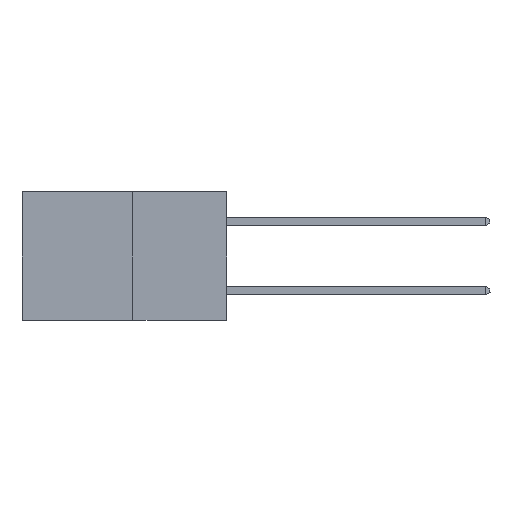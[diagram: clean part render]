
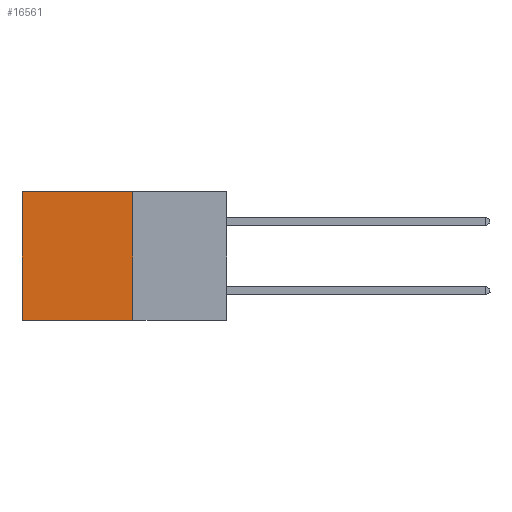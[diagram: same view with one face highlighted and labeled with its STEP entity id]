
A CAD part, left-side view. The second image highlights one B-rep face of the part: STEP entity #16561.
In plain terms, the highlighted planar face has unit normal (-1, 0, 0).
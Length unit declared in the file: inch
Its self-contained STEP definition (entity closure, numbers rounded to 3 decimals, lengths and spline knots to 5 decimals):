
#130 = FACE_OUTER_BOUND ( 'NONE', #18567, .T. ) ;
#500 = CARTESIAN_POINT ( 'NONE',  ( 0.277, 0.27, -0.37 ) ) ;
#3056 = DIRECTION ( 'NONE',  ( 0., 0., -1. ) ) ;
#3259 = EDGE_CURVE ( 'NONE', #29090, #22656, #11660, .T. ) ;
#3358 = LINE ( 'NONE', #22167, #15283 ) ;
#4871 = VECTOR ( 'NONE', #5290, 39.37008 ) ;
#5290 = DIRECTION ( 'NONE',  ( 0., 1., 0. ) ) ;
#6352 = LINE ( 'NONE', #6908, #32395 ) ;
#6908 = CARTESIAN_POINT ( 'NONE',  ( 0.277, 0.27, 0. ) ) ;
#10657 = CARTESIAN_POINT ( 'NONE',  ( 0.277, 0.27, -0.37 ) ) ;
#10675 = PLANE ( 'NONE',  #32511 ) ;
#11660 = LINE ( 'NONE', #17943, #4871 ) ;
#12040 = DIRECTION ( 'NONE',  ( 0., 1., 0. ) ) ;
#12496 = LINE ( 'NONE', #10657, #31782 ) ;
#12718 = ORIENTED_EDGE ( 'NONE', *, *, #12805, .T. ) ;
#12805 = EDGE_CURVE ( 'NONE', #28670, #32577, #6352, .T. ) ;
#15283 = VECTOR ( 'NONE', #24665, 39.37008 ) ;
#16055 = ORIENTED_EDGE ( 'NONE', *, *, #23176, .T. ) ;
#16561 = ADVANCED_FACE ( 'NONE', ( #130 ), #10675, .F. ) ;
#17910 = CARTESIAN_POINT ( 'NONE',  ( 0.277, 0.27, -0.37 ) ) ;
#17943 = CARTESIAN_POINT ( 'NONE',  ( 0.277, 0.27, -0.37 ) ) ;
#18302 = DIRECTION ( 'NONE',  ( 1., 0., 0. ) ) ;
#18567 = EDGE_LOOP ( 'NONE', ( #16055, #28684, #27943, #12718 ) ) ;
#20613 = CARTESIAN_POINT ( 'NONE',  ( 0.277, 0.27, 0. ) ) ;
#22167 = CARTESIAN_POINT ( 'NONE',  ( 0.277, 0.59, -0.37 ) ) ;
#22656 = VERTEX_POINT ( 'NONE', #27806 ) ;
#23176 = EDGE_CURVE ( 'NONE', #32577, #22656, #3358, .T. ) ;
#23518 = EDGE_CURVE ( 'NONE', #28670, #29090, #12496, .T. ) ;
#24665 = DIRECTION ( 'NONE',  ( 0., 0., -1. ) ) ;
#27806 = CARTESIAN_POINT ( 'NONE',  ( 0.277, 0.59, -0.37 ) ) ;
#27943 = ORIENTED_EDGE ( 'NONE', *, *, #23518, .F. ) ;
#28670 = VERTEX_POINT ( 'NONE', #20613 ) ;
#28684 = ORIENTED_EDGE ( 'NONE', *, *, #3259, .F. ) ;
#29090 = VERTEX_POINT ( 'NONE', #17910 ) ;
#30801 = DIRECTION ( 'NONE',  ( 0., 0., -1. ) ) ;
#31782 = VECTOR ( 'NONE', #30801, 39.37008 ) ;
#32282 = CARTESIAN_POINT ( 'NONE',  ( 0.277, 0.59, 0. ) ) ;
#32395 = VECTOR ( 'NONE', #12040, 39.37008 ) ;
#32511 = AXIS2_PLACEMENT_3D ( 'NONE', #500, #18302, #3056 ) ;
#32577 = VERTEX_POINT ( 'NONE', #32282 ) ;
